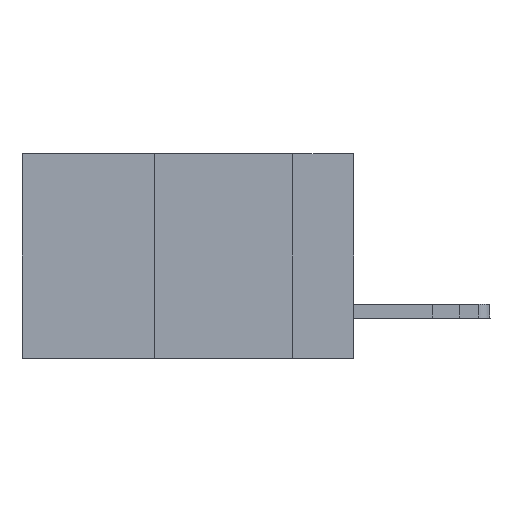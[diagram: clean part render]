
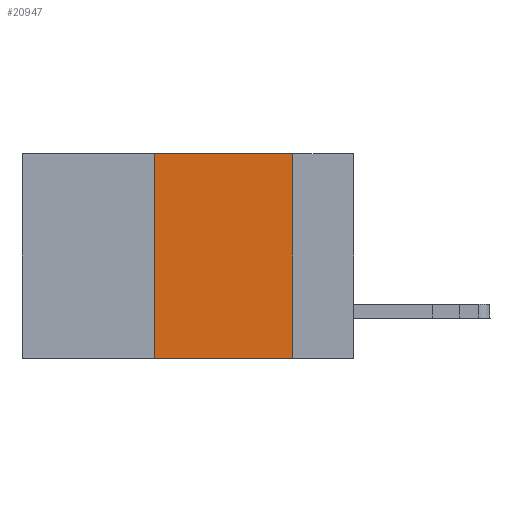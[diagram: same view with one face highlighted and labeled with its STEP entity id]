
A CAD part, left-side view. The second image highlights one B-rep face of the part: STEP entity #20947.
In plain terms, the highlighted planar face has unit normal (-1, 0, 0).
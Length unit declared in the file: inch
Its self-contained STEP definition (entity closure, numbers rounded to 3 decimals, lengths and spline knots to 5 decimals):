
#508 = EDGE_CURVE ( 'NONE', #9568, #2627, #12610, .T. ) ;
#848 = LINE ( 'NONE', #21552, #17724 ) ;
#1634 = EDGE_LOOP ( 'NONE', ( #15196, #2207, #6755, #2736 ) ) ;
#1717 = CARTESIAN_POINT ( 'NONE',  ( 0., 0.11, 0. ) ) ;
#2207 = ORIENTED_EDGE ( 'NONE', *, *, #10199, .F. ) ;
#2504 = LINE ( 'NONE', #19474, #11009 ) ;
#2627 = VERTEX_POINT ( 'NONE', #13913 ) ;
#2736 = ORIENTED_EDGE ( 'NONE', *, *, #508, .T. ) ;
#2779 = AXIS2_PLACEMENT_3D ( 'NONE', #8517, #20149, #10228 ) ;
#3400 = LINE ( 'NONE', #19955, #20704 ) ;
#3585 = VECTOR ( 'NONE', #8376, 39.37008 ) ;
#4999 = PLANE ( 'NONE',  #2779 ) ;
#6755 = ORIENTED_EDGE ( 'NONE', *, *, #14559, .F. ) ;
#8376 = DIRECTION ( 'NONE',  ( 0., -1., 0. ) ) ;
#8517 = CARTESIAN_POINT ( 'NONE',  ( 0., 0.6, 0. ) ) ;
#9364 = CARTESIAN_POINT ( 'NONE',  ( 0., 0.36, 0. ) ) ;
#9504 = CARTESIAN_POINT ( 'NONE',  ( 0., 0.6, -0.37 ) ) ;
#9568 = VERTEX_POINT ( 'NONE', #15120 ) ;
#10199 = EDGE_CURVE ( 'NONE', #18272, #11489, #3400, .T. ) ;
#10228 = DIRECTION ( 'NONE',  ( 0., 0., -1. ) ) ;
#11009 = VECTOR ( 'NONE', #14583, 39.37008 ) ;
#11489 = VERTEX_POINT ( 'NONE', #1717 ) ;
#12610 = LINE ( 'NONE', #9504, #3585 ) ;
#13399 = DIRECTION ( 'NONE',  ( 0., -1., 0. ) ) ;
#13913 = CARTESIAN_POINT ( 'NONE',  ( 0., 0.11, -0.37 ) ) ;
#14559 = EDGE_CURVE ( 'NONE', #9568, #18272, #848, .T. ) ;
#14583 = DIRECTION ( 'NONE',  ( 0., 0., -1. ) ) ;
#15052 = DIRECTION ( 'NONE',  ( 0., 0., 1. ) ) ;
#15120 = CARTESIAN_POINT ( 'NONE',  ( 0., 0.36, -0.37 ) ) ;
#15196 = ORIENTED_EDGE ( 'NONE', *, *, #16914, .F. ) ;
#16914 = EDGE_CURVE ( 'NONE', #11489, #2627, #2504, .T. ) ;
#17724 = VECTOR ( 'NONE', #15052, 39.37008 ) ;
#18272 = VERTEX_POINT ( 'NONE', #9364 ) ;
#19474 = CARTESIAN_POINT ( 'NONE',  ( 0., 0.11, 0. ) ) ;
#19955 = CARTESIAN_POINT ( 'NONE',  ( 0., 0.6, 0. ) ) ;
#20149 = DIRECTION ( 'NONE',  ( 1., 0., 0. ) ) ;
#20692 = FACE_OUTER_BOUND ( 'NONE', #1634, .T. ) ;
#20704 = VECTOR ( 'NONE', #13399, 39.37008 ) ;
#20947 = ADVANCED_FACE ( 'NONE', ( #20692 ), #4999, .F. ) ;
#21552 = CARTESIAN_POINT ( 'NONE',  ( 0., 0.36, 0. ) ) ;
